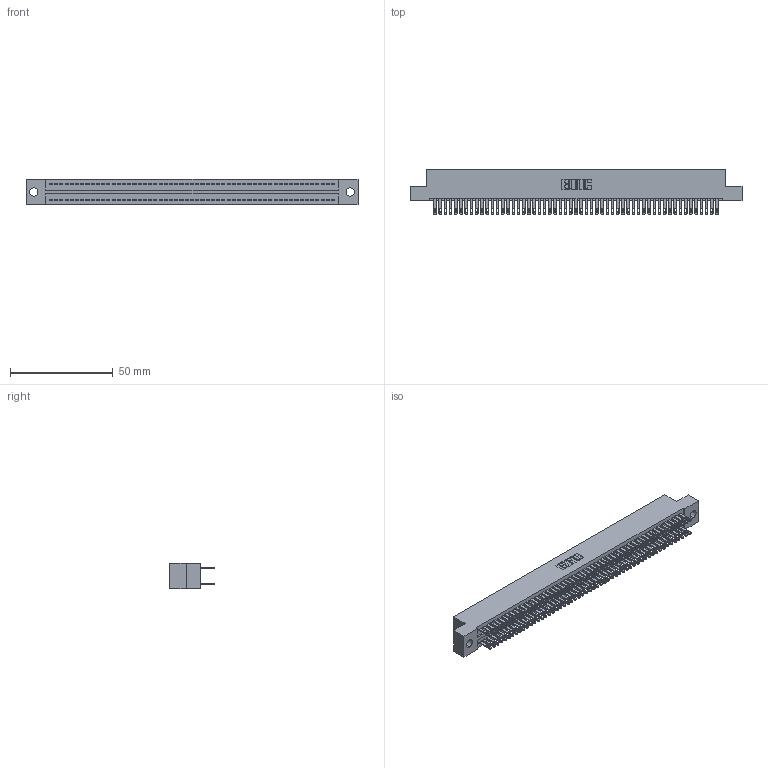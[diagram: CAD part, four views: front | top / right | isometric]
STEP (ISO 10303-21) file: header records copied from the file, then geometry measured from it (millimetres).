
FILE_DESCRIPTION (( 'STEP AP203' ), '1' );
FILE_NAME ('325-110-500-209.STEP', '2020-02-25T07:37:19', ( '' ), ( '' ), 'SwSTEP 2.0', 'SolidWorks 2016', '' );
FILE_SCHEMA (( 'CONFIG_CONTROL_DESIGN' ));
Length unit declared in the file: inch
Products named in the file (3): 325 Part_.160 TH; 325-292-001_325-293-100; 325-110-500-209
Assembly tree (111 placements, depth 2):
  325-110-500-209
    325 Part_.160 TH
    325-292-001_325-293-100  x110
Bounding box: 161.42 x 21.84 x 12.45 mm (x, y, z)
Volume: 21060.3 mm3; surface area: 26869.5 mm2
Topology: 111 solids, 111 shells, 5394 faces, 16481 edges, 10986 vertices
Faces by surface type: plane 3370, cylinder 2024
Entity records: 33635 total; most frequent: CARTESIAN_POINT 5558, ORIENTED_EDGE 5494, DIRECTION 4727, EDGE_CURVE 2747, LINE 2615, VECTOR 2615, VERTEX_POINT 1830, AXIS2_PLACEMENT_3D 1056
